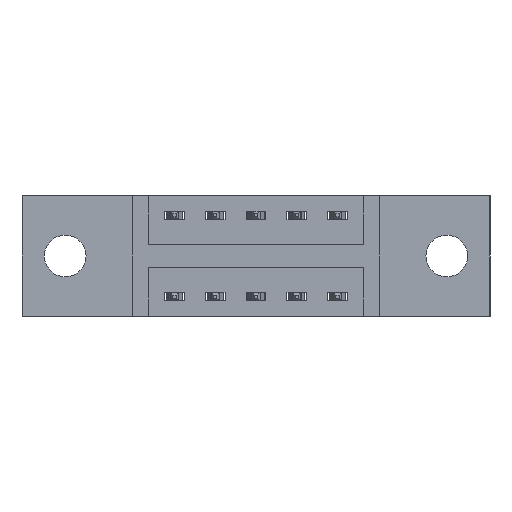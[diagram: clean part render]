
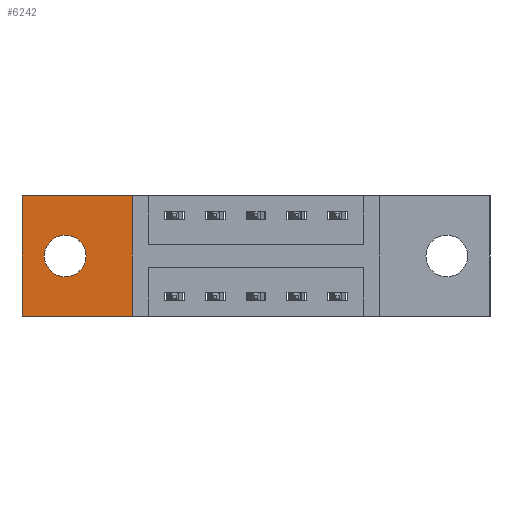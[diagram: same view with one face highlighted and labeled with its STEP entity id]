
A CAD part, front view. The second image highlights one B-rep face of the part: STEP entity #6242.
In plain terms, the highlighted planar face has unit normal (0, -1, 0).
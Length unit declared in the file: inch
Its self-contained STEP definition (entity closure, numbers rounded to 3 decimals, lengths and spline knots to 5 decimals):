
#51 = EDGE_LOOP ( 'NONE', ( #3148, #3953 ) ) ;
#211 = DIRECTION ( 'NONE',  ( 0., 0., 1. ) ) ;
#263 = ORIENTED_EDGE ( 'NONE', *, *, #7095, .T. ) ;
#319 = CIRCLE ( 'NONE', #8282, 0.064 ) ;
#398 = DIRECTION ( 'NONE',  ( 0., -1., 0. ) ) ;
#894 = VECTOR ( 'NONE', #1980, 39.37008 ) ;
#1228 = EDGE_CURVE ( 'NONE', #7433, #1252, #1287, .T. ) ;
#1252 = VERTEX_POINT ( 'NONE', #3656 ) ;
#1287 = LINE ( 'NONE', #7033, #2853 ) ;
#1319 = CARTESIAN_POINT ( 'NONE',  ( 0., 0.17, -0.37 ) ) ;
#1449 = VERTEX_POINT ( 'NONE', #4797 ) ;
#1518 = FACE_OUTER_BOUND ( 'NONE', #3752, .T. ) ;
#1543 = EDGE_CURVE ( 'NONE', #1449, #3580, #319, .T. ) ;
#1980 = DIRECTION ( 'NONE',  ( 1., 0., 0. ) ) ;
#2031 = DIRECTION ( 'NONE',  ( -1., 0., 0. ) ) ;
#2183 = AXIS2_PLACEMENT_3D ( 'NONE', #2654, #3341, #7782 ) ;
#2654 = CARTESIAN_POINT ( 'NONE',  ( 0., 0.17, -0.37 ) ) ;
#2853 = VECTOR ( 'NONE', #2031, 39.37008 ) ;
#2907 = VERTEX_POINT ( 'NONE', #4623 ) ;
#3148 = ORIENTED_EDGE ( 'NONE', *, *, #7280, .F. ) ;
#3341 = DIRECTION ( 'NONE',  ( 0., -1., 0. ) ) ;
#3491 = AXIS2_PLACEMENT_3D ( 'NONE', #4401, #398, #5096 ) ;
#3580 = VERTEX_POINT ( 'NONE', #7674 ) ;
#3656 = CARTESIAN_POINT ( 'NONE',  ( 0., 0.17, 0. ) ) ;
#3752 = EDGE_LOOP ( 'NONE', ( #263, #5871, #5276, #5577 ) ) ;
#3826 = VECTOR ( 'NONE', #4859, 39.37008 ) ;
#3953 = ORIENTED_EDGE ( 'NONE', *, *, #1543, .F. ) ;
#3966 = PLANE ( 'NONE',  #2183 ) ;
#4021 = EDGE_CURVE ( 'NONE', #2907, #7433, #7344, .T. ) ;
#4339 = CIRCLE ( 'NONE', #3491, 0.064 ) ;
#4387 = VECTOR ( 'NONE', #211, 39.37008 ) ;
#4401 = CARTESIAN_POINT ( 'NONE',  ( 0.1325, 0.17, -0.185 ) ) ;
#4428 = LINE ( 'NONE', #1319, #894 ) ;
#4623 = CARTESIAN_POINT ( 'NONE',  ( 0.3375, 0.17, -0.37 ) ) ;
#4666 = CARTESIAN_POINT ( 'NONE',  ( 0.3375, 0.17, 0. ) ) ;
#4704 = CARTESIAN_POINT ( 'NONE',  ( 0.1325, 0.17, -0.185 ) ) ;
#4797 = CARTESIAN_POINT ( 'NONE',  ( 0.1325, 0.17, -0.249 ) ) ;
#4859 = DIRECTION ( 'NONE',  ( 0., 0., -1. ) ) ;
#4884 = FACE_BOUND ( 'NONE', #51, .T. ) ;
#5096 = DIRECTION ( 'NONE',  ( 0., 0., -1. ) ) ;
#5276 = ORIENTED_EDGE ( 'NONE', *, *, #4021, .T. ) ;
#5577 = ORIENTED_EDGE ( 'NONE', *, *, #1228, .T. ) ;
#5863 = DIRECTION ( 'NONE',  ( 0., 0., -1. ) ) ;
#5871 = ORIENTED_EDGE ( 'NONE', *, *, #8163, .T. ) ;
#5965 = LINE ( 'NONE', #6729, #3826 ) ;
#6211 = CARTESIAN_POINT ( 'NONE',  ( 0.3375, 0.17, 0. ) ) ;
#6242 = ADVANCED_FACE ( 'NONE', ( #4884, #1518 ), #3966, .T. ) ;
#6366 = CARTESIAN_POINT ( 'NONE',  ( 0., 0.17, -0.37 ) ) ;
#6729 = CARTESIAN_POINT ( 'NONE',  ( 0., 0.17, 0. ) ) ;
#7033 = CARTESIAN_POINT ( 'NONE',  ( 0., 0.17, 0. ) ) ;
#7095 = EDGE_CURVE ( 'NONE', #1252, #7904, #5965, .T. ) ;
#7280 = EDGE_CURVE ( 'NONE', #3580, #1449, #4339, .T. ) ;
#7320 = DIRECTION ( 'NONE',  ( 0., -1., 0. ) ) ;
#7344 = LINE ( 'NONE', #6211, #4387 ) ;
#7433 = VERTEX_POINT ( 'NONE', #4666 ) ;
#7674 = CARTESIAN_POINT ( 'NONE',  ( 0.1325, 0.17, -0.121 ) ) ;
#7782 = DIRECTION ( 'NONE',  ( 0., 0., -1. ) ) ;
#7904 = VERTEX_POINT ( 'NONE', #6366 ) ;
#8163 = EDGE_CURVE ( 'NONE', #7904, #2907, #4428, .T. ) ;
#8282 = AXIS2_PLACEMENT_3D ( 'NONE', #4704, #7320, #5863 ) ;
